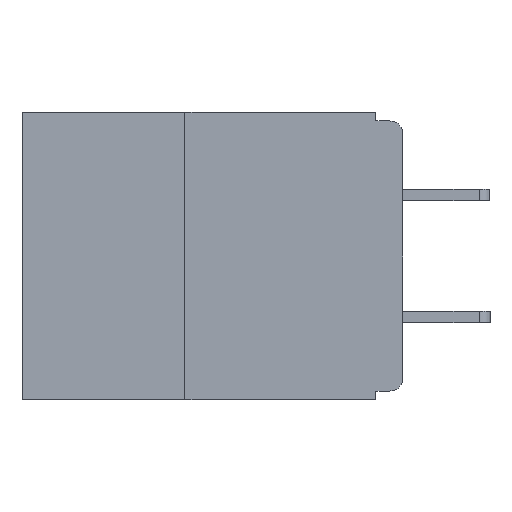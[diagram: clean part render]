
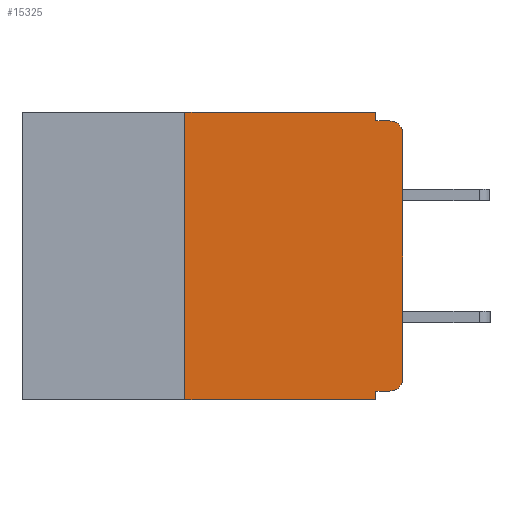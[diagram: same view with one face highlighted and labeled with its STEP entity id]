
A CAD part, left-side view. The second image highlights one B-rep face of the part: STEP entity #15325.
In plain terms, the highlighted planar face has unit normal (-1, 0, 0).
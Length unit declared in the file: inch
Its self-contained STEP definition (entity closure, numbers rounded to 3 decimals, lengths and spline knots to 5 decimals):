
#294 = EDGE_CURVE ( 'NONE', #31613, #1839, #15823, .T. ) ;
#535 = PLANE ( 'NONE',  #27958 ) ;
#1607 = EDGE_CURVE ( 'NONE', #20018, #13305, #17379, .T. ) ;
#1835 = VECTOR ( 'NONE', #2476, 39.37008 ) ;
#1839 = VERTEX_POINT ( 'NONE', #21168 ) ;
#1967 = EDGE_CURVE ( 'NONE', #5451, #31696, #21838, .T. ) ;
#1975 = ORIENTED_EDGE ( 'NONE', *, *, #294, .F. ) ;
#2476 = DIRECTION ( 'NONE',  ( 0., -1., 0. ) ) ;
#4305 = CARTESIAN_POINT ( 'NONE',  ( 0., 0.015, -0.01 ) ) ;
#4641 = DIRECTION ( 'NONE',  ( 0., 0., -1. ) ) ;
#5025 = LINE ( 'NONE', #5151, #19064 ) ;
#5151 = CARTESIAN_POINT ( 'NONE',  ( 0., 0., -0.32 ) ) ;
#5451 = VERTEX_POINT ( 'NONE', #23294 ) ;
#5733 = ORIENTED_EDGE ( 'NONE', *, *, #1607, .T. ) ;
#5901 = DIRECTION ( 'NONE',  ( 0., 0., -1. ) ) ;
#6316 = CARTESIAN_POINT ( 'NONE',  ( 0., 0.031, -0.33 ) ) ;
#6337 = ORIENTED_EDGE ( 'NONE', *, *, #1967, .T. ) ;
#6558 = CARTESIAN_POINT ( 'NONE',  ( 0., 0.031, -0.01 ) ) ;
#7839 = DIRECTION ( 'NONE',  ( 0., 1., 0. ) ) ;
#8116 = FACE_OUTER_BOUND ( 'NONE', #21148, .T. ) ;
#8849 = VECTOR ( 'NONE', #18175, 39.37008 ) ;
#8908 = VECTOR ( 'NONE', #33311, 39.37008 ) ;
#9805 = CARTESIAN_POINT ( 'NONE',  ( 0., 0., 0. ) ) ;
#10869 = EDGE_CURVE ( 'NONE', #26590, #32833, #25722, .T. ) ;
#11061 = VECTOR ( 'NONE', #30266, 39.37008 ) ;
#12071 = EDGE_CURVE ( 'NONE', #17964, #31696, #31685, .T. ) ;
#13085 = AXIS2_PLACEMENT_3D ( 'NONE', #15515, #15184, #15480 ) ;
#13305 = VERTEX_POINT ( 'NONE', #31519 ) ;
#13617 = ORIENTED_EDGE ( 'NONE', *, *, #28103, .T. ) ;
#13895 = CARTESIAN_POINT ( 'NONE',  ( 0., 0.031, 0. ) ) ;
#14265 = DIRECTION ( 'NONE',  ( 0., -1., 0. ) ) ;
#14535 = CARTESIAN_POINT ( 'NONE',  ( 0., 0.25, -0.33 ) ) ;
#15184 = DIRECTION ( 'NONE',  ( -1., 0., 0. ) ) ;
#15325 = ADVANCED_FACE ( 'NONE', ( #8116 ), #535, .F. ) ;
#15451 = EDGE_CURVE ( 'NONE', #31613, #32833, #23978, .T. ) ;
#15480 = DIRECTION ( 'NONE',  ( 0., 0., -1. ) ) ;
#15515 = CARTESIAN_POINT ( 'NONE',  ( 0., 0.015, -0.025 ) ) ;
#15823 = LINE ( 'NONE', #18204, #8849 ) ;
#15881 = LINE ( 'NONE', #23069, #8908 ) ;
#15888 = LINE ( 'NONE', #23334, #1835 ) ;
#17379 = CIRCLE ( 'NONE', #18676, 0.015 ) ;
#17785 = CARTESIAN_POINT ( 'NONE',  ( 0., 0.015, -0.32 ) ) ;
#17838 = LINE ( 'NONE', #9805, #30683 ) ;
#17964 = VERTEX_POINT ( 'NONE', #6558 ) ;
#18175 = DIRECTION ( 'NONE',  ( 0., 0., 1. ) ) ;
#18204 = CARTESIAN_POINT ( 'NONE',  ( 0., 0.25, -0.33 ) ) ;
#18676 = AXIS2_PLACEMENT_3D ( 'NONE', #30827, #30717, #30515 ) ;
#19025 = CARTESIAN_POINT ( 'NONE',  ( 0., 0.437, 0. ) ) ;
#19064 = VECTOR ( 'NONE', #7839, 39.37008 ) ;
#19491 = EDGE_CURVE ( 'NONE', #1839, #24402, #15888, .T. ) ;
#19548 = CARTESIAN_POINT ( 'NONE',  ( 0., 0.437, -0.33 ) ) ;
#20018 = VERTEX_POINT ( 'NONE', #17785 ) ;
#20358 = CARTESIAN_POINT ( 'NONE',  ( 0., 0.031, -0.33 ) ) ;
#20606 = CARTESIAN_POINT ( 'NONE',  ( 0., 0.031, -0.32 ) ) ;
#20871 = ORIENTED_EDGE ( 'NONE', *, *, #10869, .F. ) ;
#21148 = EDGE_LOOP ( 'NONE', ( #13617, #6337, #28757, #24254, #25725, #1975, #27308, #20871, #24080, #5733 ) ) ;
#21168 = CARTESIAN_POINT ( 'NONE',  ( 0., 0.25, 0. ) ) ;
#21565 = DIRECTION ( 'NONE',  ( 1., 0., 0. ) ) ;
#21838 = CIRCLE ( 'NONE', #13085, 0.015 ) ;
#23069 = CARTESIAN_POINT ( 'NONE',  ( 0., 0.031, 0. ) ) ;
#23294 = CARTESIAN_POINT ( 'NONE',  ( 0., 0., -0.025 ) ) ;
#23334 = CARTESIAN_POINT ( 'NONE',  ( 0., 0.437, 0. ) ) ;
#23978 = LINE ( 'NONE', #19548, #30785 ) ;
#24080 = ORIENTED_EDGE ( 'NONE', *, *, #32573, .F. ) ;
#24254 = ORIENTED_EDGE ( 'NONE', *, *, #26581, .F. ) ;
#24402 = VERTEX_POINT ( 'NONE', #13895 ) ;
#25722 = LINE ( 'NONE', #20358, #32489 ) ;
#25725 = ORIENTED_EDGE ( 'NONE', *, *, #19491, .F. ) ;
#26581 = EDGE_CURVE ( 'NONE', #24402, #17964, #15881, .T. ) ;
#26590 = VERTEX_POINT ( 'NONE', #20606 ) ;
#27308 = ORIENTED_EDGE ( 'NONE', *, *, #15451, .T. ) ;
#27713 = CARTESIAN_POINT ( 'NONE',  ( 0., 0., -0.01 ) ) ;
#27958 = AXIS2_PLACEMENT_3D ( 'NONE', #19025, #21565, #5901 ) ;
#27993 = DIRECTION ( 'NONE',  ( 0., 0., 1. ) ) ;
#28103 = EDGE_CURVE ( 'NONE', #13305, #5451, #17838, .T. ) ;
#28757 = ORIENTED_EDGE ( 'NONE', *, *, #12071, .F. ) ;
#30266 = DIRECTION ( 'NONE',  ( 0., -1., 0. ) ) ;
#30515 = DIRECTION ( 'NONE',  ( 0., 0., -1. ) ) ;
#30683 = VECTOR ( 'NONE', #27993, 39.37008 ) ;
#30717 = DIRECTION ( 'NONE',  ( -1., 0., 0. ) ) ;
#30785 = VECTOR ( 'NONE', #14265, 39.37008 ) ;
#30827 = CARTESIAN_POINT ( 'NONE',  ( 0., 0.015, -0.305 ) ) ;
#31519 = CARTESIAN_POINT ( 'NONE',  ( 0., 0., -0.305 ) ) ;
#31613 = VERTEX_POINT ( 'NONE', #14535 ) ;
#31685 = LINE ( 'NONE', #27713, #11061 ) ;
#31696 = VERTEX_POINT ( 'NONE', #4305 ) ;
#32489 = VECTOR ( 'NONE', #4641, 39.37008 ) ;
#32573 = EDGE_CURVE ( 'NONE', #20018, #26590, #5025, .T. ) ;
#32833 = VERTEX_POINT ( 'NONE', #6316 ) ;
#33311 = DIRECTION ( 'NONE',  ( 0., 0., -1. ) ) ;
